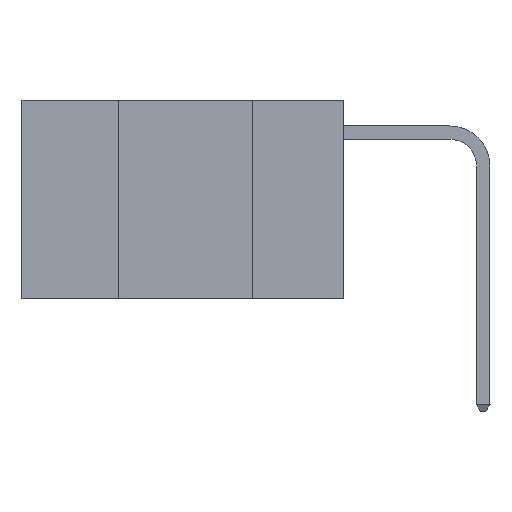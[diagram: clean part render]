
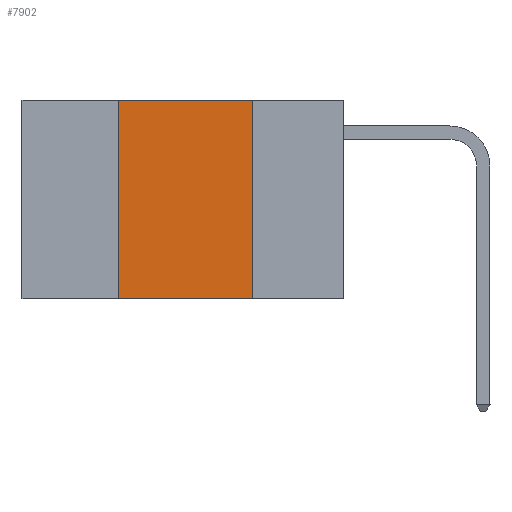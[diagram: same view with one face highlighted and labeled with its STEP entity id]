
A CAD part, left-side view. The second image highlights one B-rep face of the part: STEP entity #7902.
In plain terms, the highlighted planar face has unit normal (-1, 0, 0).
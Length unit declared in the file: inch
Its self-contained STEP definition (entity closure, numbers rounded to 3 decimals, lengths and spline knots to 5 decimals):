
#360 = VECTOR ( 'NONE', #7742, 39.37008 ) ;
#678 = CARTESIAN_POINT ( 'NONE',  ( 0., 0.17, 0. ) ) ;
#749 = FACE_OUTER_BOUND ( 'NONE', #7939, .T. ) ;
#755 = EDGE_CURVE ( 'NONE', #5092, #4973, #6640, .T. ) ;
#1393 = LINE ( 'NONE', #6998, #360 ) ;
#1528 = EDGE_CURVE ( 'NONE', #6520, #8667, #1393, .T. ) ;
#2323 = CARTESIAN_POINT ( 'NONE',  ( 0., 0.42, -0.37 ) ) ;
#3048 = ORIENTED_EDGE ( 'NONE', *, *, #6147, .T. ) ;
#3704 = EDGE_CURVE ( 'NONE', #8667, #5092, #6492, .T. ) ;
#4340 = VECTOR ( 'NONE', #7433, 39.37008 ) ;
#4758 = DIRECTION ( 'NONE',  ( 0., -1., 0. ) ) ;
#4841 = CARTESIAN_POINT ( 'NONE',  ( 0., 0.6, -0.37 ) ) ;
#4973 = VERTEX_POINT ( 'NONE', #5748 ) ;
#5092 = VERTEX_POINT ( 'NONE', #678 ) ;
#5281 = AXIS2_PLACEMENT_3D ( 'NONE', #7644, #7602, #7588 ) ;
#5748 = CARTESIAN_POINT ( 'NONE',  ( 0., 0.17, -0.37 ) ) ;
#6147 = EDGE_CURVE ( 'NONE', #6520, #4973, #8725, .T. ) ;
#6396 = VECTOR ( 'NONE', #8648, 39.37008 ) ;
#6492 = LINE ( 'NONE', #8701, #6396 ) ;
#6520 = VERTEX_POINT ( 'NONE', #2323 ) ;
#6640 = LINE ( 'NONE', #7108, #4340 ) ;
#6998 = CARTESIAN_POINT ( 'NONE',  ( 0., 0.42, 0. ) ) ;
#7108 = CARTESIAN_POINT ( 'NONE',  ( 0., 0.17, 0. ) ) ;
#7433 = DIRECTION ( 'NONE',  ( 0., 0., -1. ) ) ;
#7588 = DIRECTION ( 'NONE',  ( 0., 0., -1. ) ) ;
#7602 = DIRECTION ( 'NONE',  ( 1., 0., 0. ) ) ;
#7644 = CARTESIAN_POINT ( 'NONE',  ( 0., 0.6, 0. ) ) ;
#7742 = DIRECTION ( 'NONE',  ( 0., 0., 1. ) ) ;
#7769 = CARTESIAN_POINT ( 'NONE',  ( 0., 0.42, 0. ) ) ;
#7776 = PLANE ( 'NONE',  #5281 ) ;
#7902 = ADVANCED_FACE ( 'NONE', ( #749 ), #7776, .F. ) ;
#7930 = ORIENTED_EDGE ( 'NONE', *, *, #1528, .F. ) ;
#7939 = EDGE_LOOP ( 'NONE', ( #8023, #8036, #7930, #3048 ) ) ;
#8023 = ORIENTED_EDGE ( 'NONE', *, *, #755, .F. ) ;
#8036 = ORIENTED_EDGE ( 'NONE', *, *, #3704, .F. ) ;
#8431 = VECTOR ( 'NONE', #4758, 39.37008 ) ;
#8648 = DIRECTION ( 'NONE',  ( 0., -1., 0. ) ) ;
#8667 = VERTEX_POINT ( 'NONE', #7769 ) ;
#8701 = CARTESIAN_POINT ( 'NONE',  ( 0., 0.6, 0. ) ) ;
#8725 = LINE ( 'NONE', #4841, #8431 ) ;
